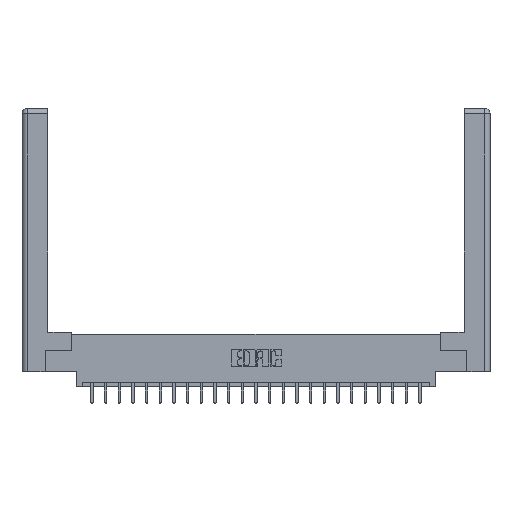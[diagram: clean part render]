
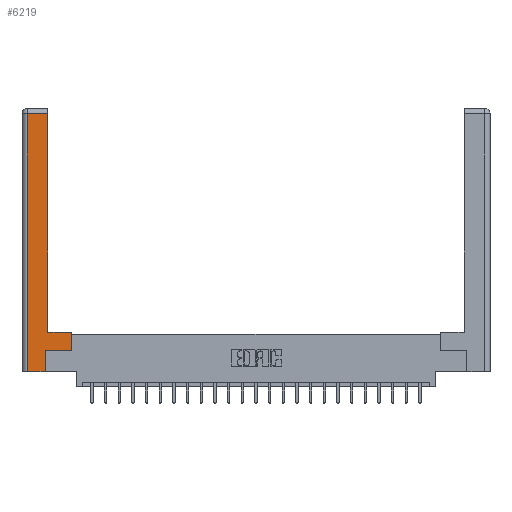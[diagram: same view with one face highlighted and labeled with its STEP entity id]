
A CAD part, top view. The second image highlights one B-rep face of the part: STEP entity #6219.
In plain terms, the highlighted planar face has unit normal (0, 0, 1).
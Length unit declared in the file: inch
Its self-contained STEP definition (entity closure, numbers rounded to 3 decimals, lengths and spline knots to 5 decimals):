
#114 = DIRECTION ( 'NONE',  ( -1., 0., 0. ) ) ;
#630 = CARTESIAN_POINT ( 'NONE',  ( 0.0615, 2.94, 0. ) ) ;
#824 = EDGE_CURVE ( 'NONE', #17825, #3929, #11096, .T. ) ;
#2292 = VERTEX_POINT ( 'NONE', #14896 ) ;
#2456 = CARTESIAN_POINT ( 'NONE',  ( 0.565, 0.245, 0. ) ) ;
#2546 = AXIS2_PLACEMENT_3D ( 'NONE', #3828, #5772, #18967 ) ;
#2561 = ORIENTED_EDGE ( 'NONE', *, *, #20728, .T. ) ;
#2798 = CARTESIAN_POINT ( 'NONE',  ( 0.295, 2.94, 0. ) ) ;
#3212 = DIRECTION ( 'NONE',  ( 0., -1., 0. ) ) ;
#3321 = CARTESIAN_POINT ( 'NONE',  ( 0.265, 0.245, 0. ) ) ;
#3352 = LINE ( 'NONE', #12313, #5166 ) ;
#3828 = CARTESIAN_POINT ( 'NONE',  ( 0., 0., 0. ) ) ;
#3842 = CARTESIAN_POINT ( 'NONE',  ( 0.565, 0.245, 0. ) ) ;
#3929 = VERTEX_POINT ( 'NONE', #2798 ) ;
#4078 = EDGE_LOOP ( 'NONE', ( #5912, #2561, #21089, #7557, #6619, #21987, #12109, #19399 ) ) ;
#4284 = DIRECTION ( 'NONE',  ( 0., 1., 0. ) ) ;
#4372 = CARTESIAN_POINT ( 'NONE',  ( 0.295, 3., 0. ) ) ;
#4594 = LINE ( 'NONE', #8532, #24067 ) ;
#4632 = DIRECTION ( 'NONE',  ( 0., 1., 0. ) ) ;
#4694 = DIRECTION ( 'NONE',  ( 1., 0., 0. ) ) ;
#5166 = VECTOR ( 'NONE', #4632, 39.37008 ) ;
#5346 = EDGE_CURVE ( 'NONE', #12350, #10386, #3352, .T. ) ;
#5772 = DIRECTION ( 'NONE',  ( 0., 0., -1. ) ) ;
#5912 = ORIENTED_EDGE ( 'NONE', *, *, #824, .T. ) ;
#6219 = ADVANCED_FACE ( 'NONE', ( #16333 ), #13272, .F. ) ;
#6268 = VECTOR ( 'NONE', #7247, 39.37008 ) ;
#6619 = ORIENTED_EDGE ( 'NONE', *, *, #13717, .T. ) ;
#7247 = DIRECTION ( 'NONE',  ( 0., 1., 0. ) ) ;
#7456 = LINE ( 'NONE', #3321, #6268 ) ;
#7557 = ORIENTED_EDGE ( 'NONE', *, *, #23726, .T. ) ;
#7836 = EDGE_CURVE ( 'NONE', #10386, #17825, #13292, .T. ) ;
#7874 = VECTOR ( 'NONE', #15113, 39.37008 ) ;
#8532 = CARTESIAN_POINT ( 'NONE',  ( 0.0615, 0., 0. ) ) ;
#8759 = DIRECTION ( 'NONE',  ( -1., 0., 0. ) ) ;
#9511 = LINE ( 'NONE', #10226, #13665 ) ;
#9934 = VECTOR ( 'NONE', #8759, 39.37008 ) ;
#10226 = CARTESIAN_POINT ( 'NONE',  ( 0.265, 0., 0. ) ) ;
#10386 = VERTEX_POINT ( 'NONE', #15294 ) ;
#10574 = CARTESIAN_POINT ( 'NONE',  ( 0.265, 0.245, 0. ) ) ;
#10640 = VECTOR ( 'NONE', #114, 39.37008 ) ;
#10792 = CARTESIAN_POINT ( 'NONE',  ( 0.295, 0.45, 0. ) ) ;
#10909 = EDGE_CURVE ( 'NONE', #18886, #15139, #4594, .T. ) ;
#11096 = LINE ( 'NONE', #4372, #18777 ) ;
#12109 = ORIENTED_EDGE ( 'NONE', *, *, #5346, .T. ) ;
#12313 = CARTESIAN_POINT ( 'NONE',  ( 0.565, 0.45, 0. ) ) ;
#12350 = VERTEX_POINT ( 'NONE', #2456 ) ;
#13272 = PLANE ( 'NONE',  #2546 ) ;
#13292 = LINE ( 'NONE', #15056, #10640 ) ;
#13665 = VECTOR ( 'NONE', #4694, 39.37008 ) ;
#13717 = EDGE_CURVE ( 'NONE', #2292, #20779, #7456, .T. ) ;
#14896 = CARTESIAN_POINT ( 'NONE',  ( 0.265, 0., 0. ) ) ;
#15056 = CARTESIAN_POINT ( 'NONE',  ( 0.295, 0.45, 0. ) ) ;
#15113 = DIRECTION ( 'NONE',  ( 1., 0., 0. ) ) ;
#15139 = VERTEX_POINT ( 'NONE', #15361 ) ;
#15270 = LINE ( 'NONE', #3842, #7874 ) ;
#15294 = CARTESIAN_POINT ( 'NONE',  ( 0.565, 0.45, 0. ) ) ;
#15361 = CARTESIAN_POINT ( 'NONE',  ( 0.0615, 0., 0. ) ) ;
#16333 = FACE_OUTER_BOUND ( 'NONE', #4078, .T. ) ;
#17825 = VERTEX_POINT ( 'NONE', #10792 ) ;
#18777 = VECTOR ( 'NONE', #4284, 39.37008 ) ;
#18886 = VERTEX_POINT ( 'NONE', #630 ) ;
#18967 = DIRECTION ( 'NONE',  ( -1., 0., 0. ) ) ;
#19115 = LINE ( 'NONE', #22017, #9934 ) ;
#19399 = ORIENTED_EDGE ( 'NONE', *, *, #7836, .T. ) ;
#20728 = EDGE_CURVE ( 'NONE', #3929, #18886, #19115, .T. ) ;
#20779 = VERTEX_POINT ( 'NONE', #10574 ) ;
#21027 = EDGE_CURVE ( 'NONE', #20779, #12350, #15270, .T. ) ;
#21089 = ORIENTED_EDGE ( 'NONE', *, *, #10909, .T. ) ;
#21987 = ORIENTED_EDGE ( 'NONE', *, *, #21027, .T. ) ;
#22017 = CARTESIAN_POINT ( 'NONE',  ( 0.0615, 2.94, 0. ) ) ;
#23726 = EDGE_CURVE ( 'NONE', #15139, #2292, #9511, .T. ) ;
#24067 = VECTOR ( 'NONE', #3212, 39.37008 ) ;
